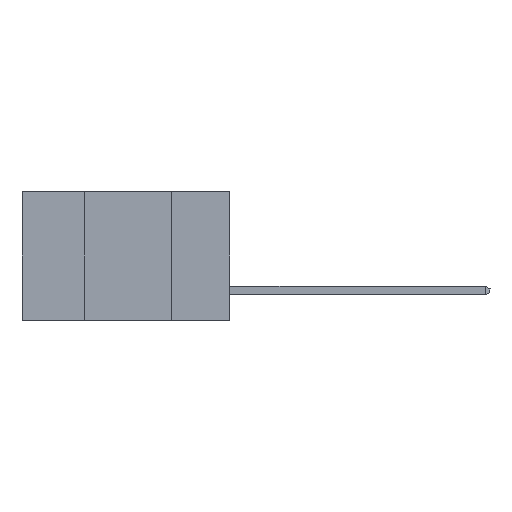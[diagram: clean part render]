
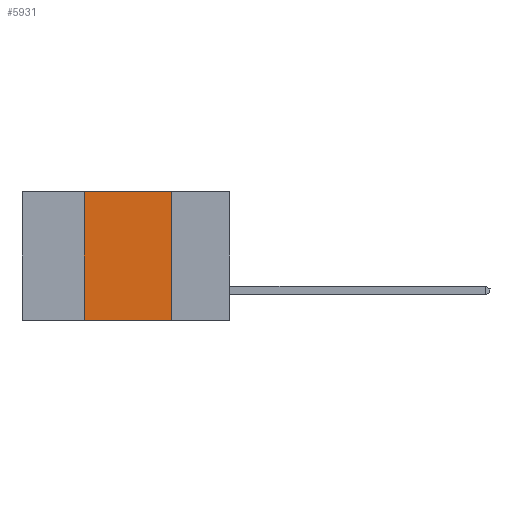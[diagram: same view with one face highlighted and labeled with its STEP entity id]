
A CAD part, left-side view. The second image highlights one B-rep face of the part: STEP entity #5931.
In plain terms, the highlighted planar face has unit normal (-1, 0, 0).
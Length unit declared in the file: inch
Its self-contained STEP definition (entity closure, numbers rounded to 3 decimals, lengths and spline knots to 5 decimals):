
#456 = CARTESIAN_POINT ( 'NONE',  ( 0., 0.42, -0.37 ) ) ;
#1145 = EDGE_CURVE ( 'NONE', #12562, #4162, #9621, .T. ) ;
#1656 = EDGE_CURVE ( 'NONE', #2914, #4162, #7190, .T. ) ;
#2002 = CARTESIAN_POINT ( 'NONE',  ( 0., 0.6, 0. ) ) ;
#2914 = VERTEX_POINT ( 'NONE', #10797 ) ;
#3099 = VECTOR ( 'NONE', #12576, 39.37008 ) ;
#3268 = EDGE_CURVE ( 'NONE', #2914, #13283, #15917, .T. ) ;
#3294 = DIRECTION ( 'NONE',  ( 1., 0., 0. ) ) ;
#4162 = VERTEX_POINT ( 'NONE', #12399 ) ;
#4708 = ORIENTED_EDGE ( 'NONE', *, *, #1656, .T. ) ;
#4860 = CARTESIAN_POINT ( 'NONE',  ( 0., 0.6, 0. ) ) ;
#5170 = EDGE_CURVE ( 'NONE', #13283, #12562, #7550, .T. ) ;
#5447 = DIRECTION ( 'NONE',  ( 0., 0., 1. ) ) ;
#5931 = ADVANCED_FACE ( 'NONE', ( #15043 ), #16763, .F. ) ;
#6550 = EDGE_LOOP ( 'NONE', ( #14173, #8754, #15129, #4708 ) ) ;
#7190 = LINE ( 'NONE', #12656, #3099 ) ;
#7335 = VECTOR ( 'NONE', #5447, 39.37008 ) ;
#7550 = LINE ( 'NONE', #4860, #12619 ) ;
#8248 = DIRECTION ( 'NONE',  ( 0., 0., -1. ) ) ;
#8527 = CARTESIAN_POINT ( 'NONE',  ( 0., 0.42, 0. ) ) ;
#8754 = ORIENTED_EDGE ( 'NONE', *, *, #5170, .F. ) ;
#9621 = LINE ( 'NONE', #12097, #16370 ) ;
#9999 = DIRECTION ( 'NONE',  ( 0., 0., -1. ) ) ;
#10797 = CARTESIAN_POINT ( 'NONE',  ( 0., 0.42, -0.37 ) ) ;
#11652 = DIRECTION ( 'NONE',  ( 0., -1., 0. ) ) ;
#12097 = CARTESIAN_POINT ( 'NONE',  ( 0., 0.17, -0.37 ) ) ;
#12399 = CARTESIAN_POINT ( 'NONE',  ( 0., 0.17, -0.37 ) ) ;
#12562 = VERTEX_POINT ( 'NONE', #14350 ) ;
#12576 = DIRECTION ( 'NONE',  ( 0., -1., 0. ) ) ;
#12619 = VECTOR ( 'NONE', #11652, 39.37008 ) ;
#12656 = CARTESIAN_POINT ( 'NONE',  ( 0., 0.6, -0.37 ) ) ;
#13283 = VERTEX_POINT ( 'NONE', #8527 ) ;
#14173 = ORIENTED_EDGE ( 'NONE', *, *, #1145, .F. ) ;
#14350 = CARTESIAN_POINT ( 'NONE',  ( 0., 0.17, 0. ) ) ;
#14722 = AXIS2_PLACEMENT_3D ( 'NONE', #2002, #3294, #9999 ) ;
#15043 = FACE_OUTER_BOUND ( 'NONE', #6550, .T. ) ;
#15129 = ORIENTED_EDGE ( 'NONE', *, *, #3268, .F. ) ;
#15917 = LINE ( 'NONE', #456, #7335 ) ;
#16370 = VECTOR ( 'NONE', #8248, 39.37008 ) ;
#16763 = PLANE ( 'NONE',  #14722 ) ;
